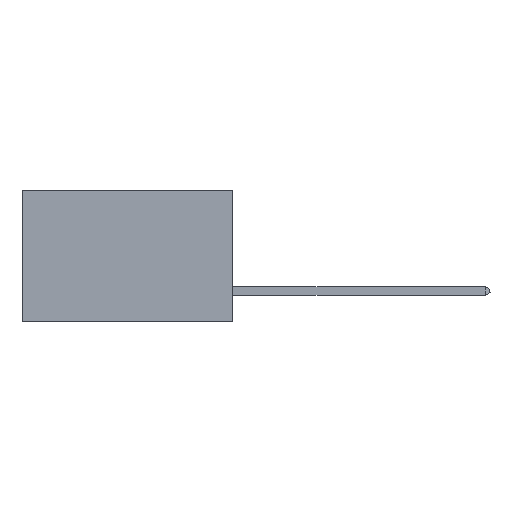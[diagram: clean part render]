
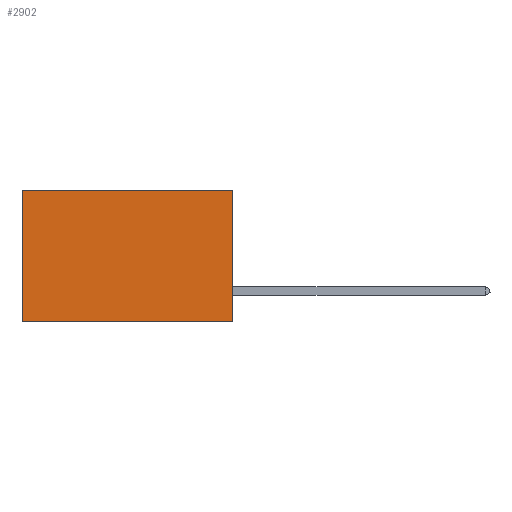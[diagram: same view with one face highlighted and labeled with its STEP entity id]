
A CAD part, left-side view. The second image highlights one B-rep face of the part: STEP entity #2902.
In plain terms, the highlighted planar face has unit normal (-1, 0, 0).
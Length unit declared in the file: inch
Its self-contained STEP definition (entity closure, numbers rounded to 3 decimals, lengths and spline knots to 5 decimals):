
#146 = DIRECTION ( 'NONE',  ( 0., 1., 0. ) ) ;
#270 = DIRECTION ( 'NONE',  ( 0., 0., -1. ) ) ;
#479 = DIRECTION ( 'NONE',  ( 1., 0., 0. ) ) ;
#718 = EDGE_CURVE ( 'NONE', #10307, #12650, #5769, .T. ) ;
#777 = AXIS2_PLACEMENT_3D ( 'NONE', #12034, #479, #14167 ) ;
#1427 = DIRECTION ( 'NONE',  ( 0., 1., 0. ) ) ;
#1946 = EDGE_LOOP ( 'NONE', ( #14741, #3794, #10323, #6061 ) ) ;
#2902 = ADVANCED_FACE ( 'NONE', ( #9457 ), #4040, .F. ) ;
#3182 = DIRECTION ( 'NONE',  ( 0., 0., -1. ) ) ;
#3794 = ORIENTED_EDGE ( 'NONE', *, *, #718, .F. ) ;
#4040 = PLANE ( 'NONE',  #777 ) ;
#4240 = CARTESIAN_POINT ( 'NONE',  ( 0.2875, 0., -0.375 ) ) ;
#4464 = EDGE_CURVE ( 'NONE', #7830, #12650, #12576, .T. ) ;
#4643 = VECTOR ( 'NONE', #146, 39.37008 ) ;
#5341 = VECTOR ( 'NONE', #3182, 39.37008 ) ;
#5431 = CARTESIAN_POINT ( 'NONE',  ( 0.2875, 0., 0. ) ) ;
#5769 = LINE ( 'NONE', #10530, #6673 ) ;
#6019 = VERTEX_POINT ( 'NONE', #5431 ) ;
#6061 = ORIENTED_EDGE ( 'NONE', *, *, #12473, .T. ) ;
#6673 = VECTOR ( 'NONE', #1427, 39.37008 ) ;
#7027 = CARTESIAN_POINT ( 'NONE',  ( 0.2875, 0., 0. ) ) ;
#7246 = CARTESIAN_POINT ( 'NONE',  ( 0.2875, 0.6, 0. ) ) ;
#7667 = LINE ( 'NONE', #4240, #5341 ) ;
#7830 = VERTEX_POINT ( 'NONE', #7246 ) ;
#8170 = CARTESIAN_POINT ( 'NONE',  ( 0.2875, 0., -0.375 ) ) ;
#9314 = CARTESIAN_POINT ( 'NONE',  ( 0.2875, 0.6, -0.375 ) ) ;
#9457 = FACE_OUTER_BOUND ( 'NONE', #1946, .T. ) ;
#9895 = CARTESIAN_POINT ( 'NONE',  ( 0.2875, 0.6, -0.375 ) ) ;
#10307 = VERTEX_POINT ( 'NONE', #8170 ) ;
#10323 = ORIENTED_EDGE ( 'NONE', *, *, #13378, .F. ) ;
#10530 = CARTESIAN_POINT ( 'NONE',  ( 0.2875, 0., -0.375 ) ) ;
#11502 = VECTOR ( 'NONE', #270, 39.37008 ) ;
#12034 = CARTESIAN_POINT ( 'NONE',  ( 0.2875, 0., -0.375 ) ) ;
#12473 = EDGE_CURVE ( 'NONE', #6019, #7830, #13216, .T. ) ;
#12576 = LINE ( 'NONE', #9314, #11502 ) ;
#12650 = VERTEX_POINT ( 'NONE', #9895 ) ;
#13216 = LINE ( 'NONE', #7027, #4643 ) ;
#13378 = EDGE_CURVE ( 'NONE', #6019, #10307, #7667, .T. ) ;
#14167 = DIRECTION ( 'NONE',  ( 0., 0., -1. ) ) ;
#14741 = ORIENTED_EDGE ( 'NONE', *, *, #4464, .T. ) ;
